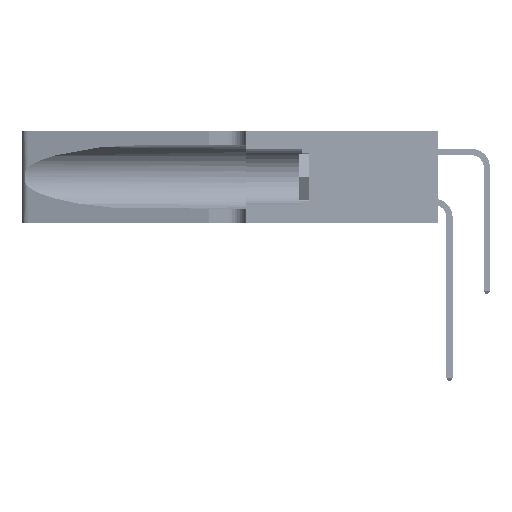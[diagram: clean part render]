
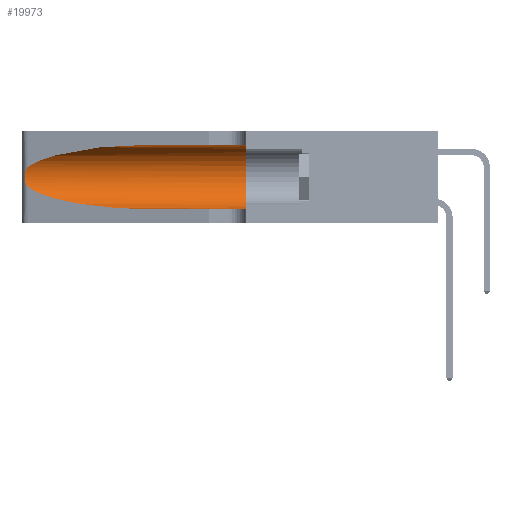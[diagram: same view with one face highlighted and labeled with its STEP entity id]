
A CAD part, left-side view. The second image highlights one B-rep face of the part: STEP entity #19973.
In plain terms, the highlighted cylindrical face has radius 3.308 mm (diameter 6.617 mm), a partial arc.
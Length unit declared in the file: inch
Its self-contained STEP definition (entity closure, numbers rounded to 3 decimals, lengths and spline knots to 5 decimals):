
#445 = CARTESIAN_POINT ( 'NONE',  ( 0.25487, 1.22718, 0.14631 ) ) ;
#1096 = LINE ( 'NONE', #3435, #16047 ) ;
#1144 = CARTESIAN_POINT ( 'NONE',  ( 0.25639, 1.23184, 0.21858 ) ) ;
#2955 = ORIENTED_EDGE ( 'NONE', *, *, #31475, .F. ) ;
#3397 = CARTESIAN_POINT ( 'NONE',  ( 0.2373, 1.15595, 0.08982 ) ) ;
#3435 = CARTESIAN_POINT ( 'NONE',  ( 0.1305, 1.61858, 0.05475 ) ) ;
#3611 = FACE_OUTER_BOUND ( 'NONE', #26952, .T. ) ;
#4088 = EDGE_CURVE ( 'NONE', #18635, #4354, #23911, .T. ) ;
#4331 = CARTESIAN_POINT ( 'NONE',  ( 0.1305, 1.61858, 0.185 ) ) ;
#4354 = VERTEX_POINT ( 'NONE', #41267 ) ;
#4498 = CARTESIAN_POINT ( 'NONE',  ( 0.25487, 1.22718, 0.22369 ) ) ;
#5171 = CARTESIAN_POINT ( 'NONE',  ( 0.25789, 1.23486, 0.15765 ) ) ;
#7026 = ORIENTED_EDGE ( 'NONE', *, *, #10402, .T. ) ;
#8995 = CARTESIAN_POINT ( 'NONE',  ( 0.25787, 1.23484, 0.2124 ) ) ;
#10402 = EDGE_CURVE ( 'NONE', #25907, #29803, #18241, .T. ) ;
#11801 = DIRECTION ( 'NONE',  ( 0., 0., -1. ) ) ;
#12026 = CARTESIAN_POINT ( 'NONE',  ( 0.1305, 1.61858, 0.31525 ) ) ;
#14624 = ORIENTED_EDGE ( 'NONE', *, *, #29892, .T. ) ;
#15623 = LINE ( 'NONE', #12026, #43304 ) ;
#16047 = VECTOR ( 'NONE', #36204, 39.37008 ) ;
#16279 = CARTESIAN_POINT ( 'NONE',  ( 0.25487, 1.22718, 0.22369 ) ) ;
#16614 = DIRECTION ( 'NONE',  ( 0., 0., 1. ) ) ;
#16663 = CARTESIAN_POINT ( 'NONE',  ( 0.25555, 1.22994, 0.2215 ) ) ;
#16687 = CARTESIAN_POINT ( 'NONE',  ( 0.18966, 0.96281, 0.31525 ) ) ;
#17012 = CARTESIAN_POINT ( 'NONE',  ( 0.26075, 1.23896, 0.178 ) ) ;
#18241 = B_SPLINE_CURVE_WITH_KNOTS ( 'NONE', 3,
 ( #25127, #16663, #1144, #8995, #36375, #41096, #32522, #17012, #49152, #29151, #5171, #44433, #48456, #445 ),
 .UNSPECIFIED., .F., .F.,
 ( 4, 2, 2, 2, 2, 2, 4 ),
 ( 0., 0.00027, 0.00053, 0.00107, 0.0016, 0.00187, 0.00214 ),
 .UNSPECIFIED. ) ;
#18635 = VERTEX_POINT ( 'NONE', #23702 ) ;
#19268 = CARTESIAN_POINT ( 'NONE',  ( 0.1305, 0.72297, 0.05475 ) ) ;
#19487 = DIRECTION ( 'NONE',  ( 0., -1., 0. ) ) ;
#19973 = ADVANCED_FACE ( 'NONE', ( #3611 ), #38710, .F. ) ;
#21367 = CARTESIAN_POINT ( 'NONE',  ( 0.1305, 0.72297, 0.31525 ) ) ;
#21865 = VERTEX_POINT ( 'NONE', #26043 ) ;
#22175 = EDGE_CURVE ( 'NONE', #31073, #25907, #45318, .T. ) ;
#22988 = CARTESIAN_POINT ( 'NONE',  ( 0.25487, 1.22718, 0.14631 ) ) ;
#23354 = AXIS2_PLACEMENT_3D ( 'NONE', #4331, #19487, #11801 ) ;
#23702 = CARTESIAN_POINT ( 'NONE',  ( 0.1305, 0.35, 0.31525 ) ) ;
#23911 = CIRCLE ( 'NONE', #42380, 0.13025 ) ;
#25127 = CARTESIAN_POINT ( 'NONE',  ( 0.25487, 1.22718, 0.22369 ) ) ;
#25907 = VERTEX_POINT ( 'NONE', #16279 ) ;
#26043 = CARTESIAN_POINT ( 'NONE',  ( 0.1305, 0.72297, 0.05475 ) ) ;
#26952 = EDGE_LOOP ( 'NONE', ( #42319, #7026, #46229, #14624, #33373, #2955 ) ) ;
#28485 = CARTESIAN_POINT ( 'NONE',  ( 0.2373, 1.15595, 0.28018 ) ) ;
#28922 = CARTESIAN_POINT ( 'NONE',  ( 0.1305, 0.35, 0.185 ) ) ;
#29151 = CARTESIAN_POINT ( 'NONE',  ( 0.25856, 1.23593, 0.16098 ) ) ;
#29803 = VERTEX_POINT ( 'NONE', #43567 ) ;
#29892 = EDGE_CURVE ( 'NONE', #21865, #4354, #1096, .T. ) ;
#31073 = VERTEX_POINT ( 'NONE', #21367 ) ;
#31475 = EDGE_CURVE ( 'NONE', #31073, #18635, #15623, .T. ) ;
#31552 = DIRECTION ( 'NONE',  ( 0., -1., 0. ) ) ;
#32522 = CARTESIAN_POINT ( 'NONE',  ( 0.26075, 1.23896, 0.19203 ) ) ;
#33373 = ORIENTED_EDGE ( 'NONE', *, *, #4088, .F. ) ;
#36204 = DIRECTION ( 'NONE',  ( 0., -1., 0. ) ) ;
#36375 = CARTESIAN_POINT ( 'NONE',  ( 0.25854, 1.2359, 0.20912 ) ) ;
#38548 =( BOUNDED_CURVE ( )  B_SPLINE_CURVE ( 3, ( #22988, #3397, #50696, #19268 ),
 .UNSPECIFIED., .F., .T. ) 
 B_SPLINE_CURVE_WITH_KNOTS ( ( 4, 4 ),
 ( 3.44316, 4.71239 ),
 .UNSPECIFIED. ) 
 CURVE ( )  GEOMETRIC_REPRESENTATION_ITEM ( )  RATIONAL_B_SPLINE_CURVE ( ( 1., 0.87, 0.87, 1. ) ) 
 REPRESENTATION_ITEM ( '' )  );
#38710 = CYLINDRICAL_SURFACE ( 'NONE', #23354, 0.13025 ) ;
#40696 = DIRECTION ( 'NONE',  ( 0., 1., 0. ) ) ;
#41096 = CARTESIAN_POINT ( 'NONE',  ( 0.26018, 1.23835, 0.19895 ) ) ;
#41267 = CARTESIAN_POINT ( 'NONE',  ( 0.1305, 0.35, 0.05475 ) ) ;
#42319 = ORIENTED_EDGE ( 'NONE', *, *, #22175, .T. ) ;
#42380 = AXIS2_PLACEMENT_3D ( 'NONE', #28922, #40696, #16614 ) ;
#42432 = EDGE_CURVE ( 'NONE', #29803, #21865, #38548, .T. ) ;
#43304 = VECTOR ( 'NONE', #31552, 39.37008 ) ;
#43567 = CARTESIAN_POINT ( 'NONE',  ( 0.25487, 1.22718, 0.14631 ) ) ;
#44433 = CARTESIAN_POINT ( 'NONE',  ( 0.25639, 1.23186, 0.15144 ) ) ;
#44823 = CARTESIAN_POINT ( 'NONE',  ( 0.1305, 0.72297, 0.31525 ) ) ;
#45318 =( BOUNDED_CURVE ( )  B_SPLINE_CURVE ( 3, ( #44823, #16687, #28485, #4498 ),
 .UNSPECIFIED., .F., .F. ) 
 B_SPLINE_CURVE_WITH_KNOTS ( ( 4, 4 ),
 ( 1.5708, 2.84003 ),
 .UNSPECIFIED. ) 
 CURVE ( )  GEOMETRIC_REPRESENTATION_ITEM ( )  RATIONAL_B_SPLINE_CURVE ( ( 1., 0.87, 0.87, 1. ) ) 
 REPRESENTATION_ITEM ( '' )  );
#46229 = ORIENTED_EDGE ( 'NONE', *, *, #42432, .T. ) ;
#48456 = CARTESIAN_POINT ( 'NONE',  ( 0.25555, 1.22993, 0.14849 ) ) ;
#49152 = CARTESIAN_POINT ( 'NONE',  ( 0.26017, 1.23833, 0.17102 ) ) ;
#50696 = CARTESIAN_POINT ( 'NONE',  ( 0.18966, 0.96281, 0.05475 ) ) ;
